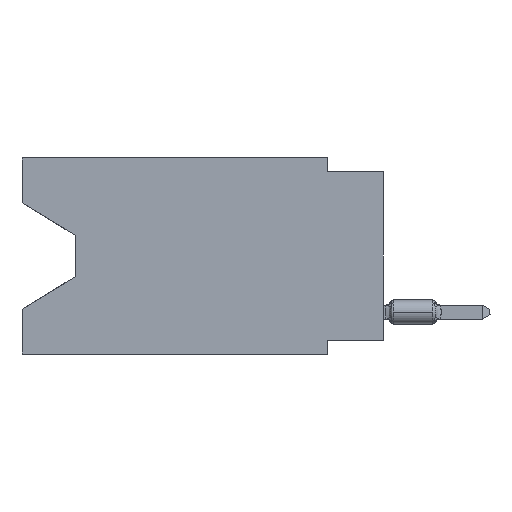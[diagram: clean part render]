
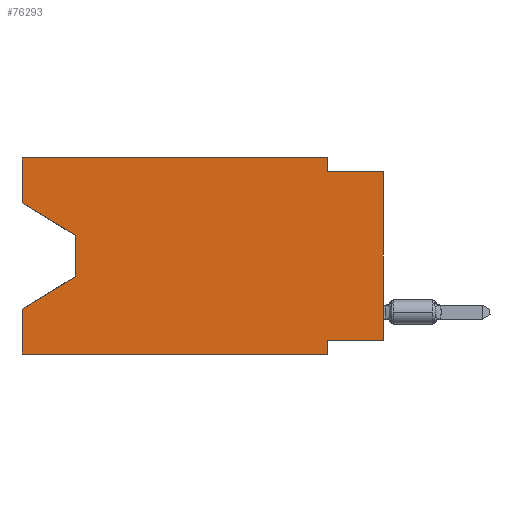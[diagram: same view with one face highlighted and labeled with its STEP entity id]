
A CAD part, left-side view. The second image highlights one B-rep face of the part: STEP entity #76293.
In plain terms, the highlighted planar face has unit normal (-1, 0, 0).
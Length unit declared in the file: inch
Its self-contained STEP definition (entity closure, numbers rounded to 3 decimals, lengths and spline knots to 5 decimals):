
#1186 = EDGE_CURVE ( 'NONE', #27831, #67969, #45344, .T. ) ;
#2543 = CARTESIAN_POINT ( 'NONE',  ( 0., 0.645, -0.35 ) ) ;
#3081 = DIRECTION ( 'NONE',  ( 0., -1., 0. ) ) ;
#3380 = DIRECTION ( 'NONE',  ( 0., -0.855, -0.519 ) ) ;
#3872 = EDGE_CURVE ( 'NONE', #98751, #23819, #7020, .T. ) ;
#4658 = ORIENTED_EDGE ( 'NONE', *, *, #93198, .T. ) ;
#7020 = LINE ( 'NONE', #38972, #10260 ) ;
#8986 = VECTOR ( 'NONE', #88153, 39.37008 ) ;
#9711 = LINE ( 'NONE', #42698, #48258 ) ;
#10260 = VECTOR ( 'NONE', #65330, 39.37008 ) ;
#10780 = EDGE_LOOP ( 'NONE', ( #65460, #33624, #94384, #102664, #4658, #99878, #106770, #96235, #81930, #19495, #41536, #81136 ) ) ;
#11728 = CARTESIAN_POINT ( 'NONE',  ( 0., 0.645, 0. ) ) ;
#11913 = VERTEX_POINT ( 'NONE', #77301 ) ;
#12654 = CARTESIAN_POINT ( 'NONE',  ( 0., 0., 0. ) ) ;
#13750 = LINE ( 'NONE', #12654, #26485 ) ;
#14467 = CARTESIAN_POINT ( 'NONE',  ( 0., 0.55, -0.212 ) ) ;
#19495 = ORIENTED_EDGE ( 'NONE', *, *, #27986, .F. ) ;
#20064 = DIRECTION ( 'NONE',  ( 0., 0., 1. ) ) ;
#21993 = VERTEX_POINT ( 'NONE', #35130 ) ;
#23819 = VERTEX_POINT ( 'NONE', #50932 ) ;
#24844 = LINE ( 'NONE', #73809, #44165 ) ;
#25236 = PLANE ( 'NONE',  #86060 ) ;
#26485 = VECTOR ( 'NONE', #46186, 39.37008 ) ;
#26801 = CARTESIAN_POINT ( 'NONE',  ( 0., 0.1, -0.35 ) ) ;
#27831 = VERTEX_POINT ( 'NONE', #29452 ) ;
#27986 = EDGE_CURVE ( 'NONE', #58713, #93228, #64085, .T. ) ;
#29452 = CARTESIAN_POINT ( 'NONE',  ( 0., 0.645, -0.35 ) ) ;
#31009 = VERTEX_POINT ( 'NONE', #43758 ) ;
#31319 = LINE ( 'NONE', #98402, #41831 ) ;
#32398 = DIRECTION ( 'NONE',  ( 0., 0., -1. ) ) ;
#33491 = FACE_OUTER_BOUND ( 'NONE', #10780, .T. ) ;
#33624 = ORIENTED_EDGE ( 'NONE', *, *, #36013, .T. ) ;
#35130 = CARTESIAN_POINT ( 'NONE',  ( 0., 0.645, -0.08025 ) ) ;
#35897 = VECTOR ( 'NONE', #45260, 39.37008 ) ;
#36013 = EDGE_CURVE ( 'NONE', #68264, #85478, #31319, .T. ) ;
#38662 = LINE ( 'NONE', #14467, #8986 ) ;
#38972 = CARTESIAN_POINT ( 'NONE',  ( 0., 0., -0.325 ) ) ;
#39075 = EDGE_CURVE ( 'NONE', #98751, #11913, #13750, .T. ) ;
#41536 = ORIENTED_EDGE ( 'NONE', *, *, #48344, .F. ) ;
#41831 = VECTOR ( 'NONE', #32398, 39.37008 ) ;
#42698 = CARTESIAN_POINT ( 'NONE',  ( 0., 0.1, -0.35 ) ) ;
#43331 = CARTESIAN_POINT ( 'NONE',  ( 0., 0.645, -0.26975 ) ) ;
#43758 = CARTESIAN_POINT ( 'NONE',  ( 0., 0.645, 0. ) ) ;
#44165 = VECTOR ( 'NONE', #83669, 39.37008 ) ;
#45260 = DIRECTION ( 'NONE',  ( 0., -1., 0. ) ) ;
#45344 = LINE ( 'NONE', #104749, #97249 ) ;
#45432 = CARTESIAN_POINT ( 'NONE',  ( 0., 0.645, 0. ) ) ;
#46186 = DIRECTION ( 'NONE',  ( 0., 0., 1. ) ) ;
#48192 = VECTOR ( 'NONE', #72869, 39.37008 ) ;
#48258 = VECTOR ( 'NONE', #76222, 39.37008 ) ;
#48344 = EDGE_CURVE ( 'NONE', #31009, #58713, #87040, .T. ) ;
#50932 = CARTESIAN_POINT ( 'NONE',  ( 0., 0.1, -0.325 ) ) ;
#50942 = LINE ( 'NONE', #2543, #55320 ) ;
#53140 = DIRECTION ( 'NONE',  ( 0., 0., 1. ) ) ;
#55176 = VECTOR ( 'NONE', #3380, 39.37008 ) ;
#55320 = VECTOR ( 'NONE', #3081, 39.37008 ) ;
#57178 = CARTESIAN_POINT ( 'NONE',  ( 0., 0.645, 0. ) ) ;
#58713 = VERTEX_POINT ( 'NONE', #93628 ) ;
#64085 = LINE ( 'NONE', #84745, #48192 ) ;
#65090 = EDGE_CURVE ( 'NONE', #21993, #68264, #79807, .T. ) ;
#65330 = DIRECTION ( 'NONE',  ( 0., 1., 0. ) ) ;
#65460 = ORIENTED_EDGE ( 'NONE', *, *, #65090, .T. ) ;
#67969 = VERTEX_POINT ( 'NONE', #43331 ) ;
#68264 = VERTEX_POINT ( 'NONE', #101362 ) ;
#70709 = CARTESIAN_POINT ( 'NONE',  ( 0., 0.1, -0.025 ) ) ;
#72869 = DIRECTION ( 'NONE',  ( 0., 0., -1. ) ) ;
#73809 = CARTESIAN_POINT ( 'NONE',  ( 0., 0., -0.025 ) ) ;
#76222 = DIRECTION ( 'NONE',  ( 0., 0., -1. ) ) ;
#76293 = ADVANCED_FACE ( 'NONE', ( #33491 ), #25236, .F. ) ;
#77010 = EDGE_CURVE ( 'NONE', #85478, #67969, #38662, .T. ) ;
#77138 = EDGE_CURVE ( 'NONE', #93228, #11913, #24844, .T. ) ;
#77301 = CARTESIAN_POINT ( 'NONE',  ( 0., 0., -0.025 ) ) ;
#79715 = EDGE_CURVE ( 'NONE', #21993, #31009, #85574, .T. ) ;
#79807 = LINE ( 'NONE', #105121, #55176 ) ;
#81136 = ORIENTED_EDGE ( 'NONE', *, *, #79715, .F. ) ;
#81930 = ORIENTED_EDGE ( 'NONE', *, *, #77138, .F. ) ;
#82983 = DIRECTION ( 'NONE',  ( 1., 0., 0. ) ) ;
#83669 = DIRECTION ( 'NONE',  ( 0., -1., 0. ) ) ;
#83940 = VERTEX_POINT ( 'NONE', #26801 ) ;
#84745 = CARTESIAN_POINT ( 'NONE',  ( 0., 0.1, 0. ) ) ;
#84900 = CARTESIAN_POINT ( 'NONE',  ( 0., 0., -0.325 ) ) ;
#85478 = VERTEX_POINT ( 'NONE', #88915 ) ;
#85574 = LINE ( 'NONE', #45432, #103986 ) ;
#86060 = AXIS2_PLACEMENT_3D ( 'NONE', #57178, #82983, #92328 ) ;
#87040 = LINE ( 'NONE', #11728, #35897 ) ;
#88153 = DIRECTION ( 'NONE',  ( 0., 0.855, -0.519 ) ) ;
#88915 = CARTESIAN_POINT ( 'NONE',  ( 0., 0.55, -0.212 ) ) ;
#92328 = DIRECTION ( 'NONE',  ( 0., 0., -1. ) ) ;
#93131 = EDGE_CURVE ( 'NONE', #23819, #83940, #9711, .T. ) ;
#93198 = EDGE_CURVE ( 'NONE', #27831, #83940, #50942, .T. ) ;
#93228 = VERTEX_POINT ( 'NONE', #70709 ) ;
#93628 = CARTESIAN_POINT ( 'NONE',  ( 0., 0.1, 0. ) ) ;
#94384 = ORIENTED_EDGE ( 'NONE', *, *, #77010, .T. ) ;
#96235 = ORIENTED_EDGE ( 'NONE', *, *, #39075, .T. ) ;
#97249 = VECTOR ( 'NONE', #20064, 39.37008 ) ;
#98402 = CARTESIAN_POINT ( 'NONE',  ( 0., 0.55, -0.138 ) ) ;
#98751 = VERTEX_POINT ( 'NONE', #84900 ) ;
#99878 = ORIENTED_EDGE ( 'NONE', *, *, #93131, .F. ) ;
#101362 = CARTESIAN_POINT ( 'NONE',  ( 0., 0.55, -0.138 ) ) ;
#102664 = ORIENTED_EDGE ( 'NONE', *, *, #1186, .F. ) ;
#103986 = VECTOR ( 'NONE', #53140, 39.37008 ) ;
#104749 = CARTESIAN_POINT ( 'NONE',  ( 0., 0.645, 0. ) ) ;
#105121 = CARTESIAN_POINT ( 'NONE',  ( 0., 0.645, -0.08025 ) ) ;
#106770 = ORIENTED_EDGE ( 'NONE', *, *, #3872, .F. ) ;
